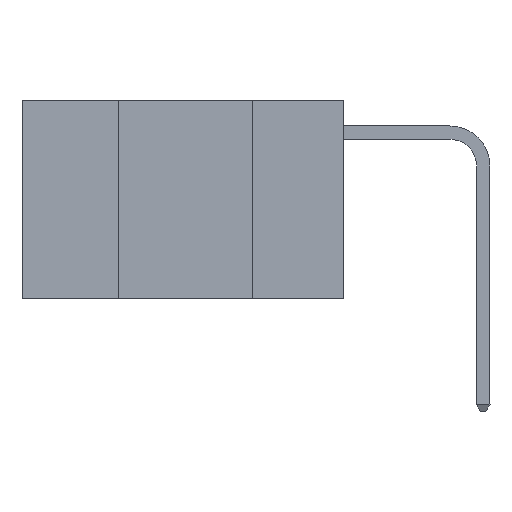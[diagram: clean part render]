
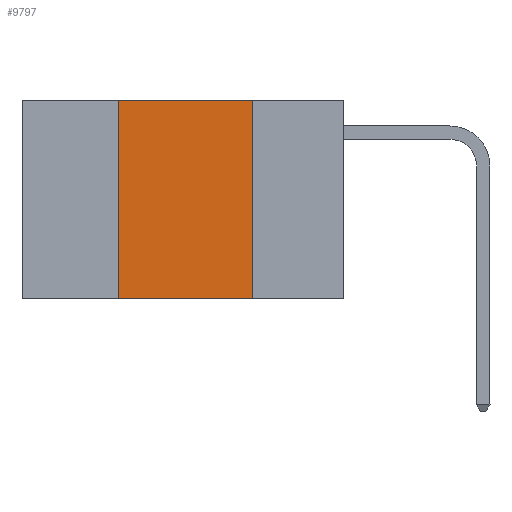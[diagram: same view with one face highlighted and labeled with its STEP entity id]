
A CAD part, left-side view. The second image highlights one B-rep face of the part: STEP entity #9797.
In plain terms, the highlighted planar face has unit normal (-1, 0, 0).
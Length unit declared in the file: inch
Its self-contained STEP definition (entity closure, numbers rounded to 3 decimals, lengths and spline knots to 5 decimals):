
#2934 = VECTOR ( 'NONE', #3183, 39.37008 ) ;
#3183 = DIRECTION ( 'NONE',  ( 0., 0., -1. ) ) ;
#4723 = ORIENTED_EDGE ( 'NONE', *, *, #18762, .F. ) ;
#4965 = ORIENTED_EDGE ( 'NONE', *, *, #8023, .F. ) ;
#5077 = CARTESIAN_POINT ( 'NONE',  ( 0., 0.6, -0.37 ) ) ;
#5193 = DIRECTION ( 'NONE',  ( 1., 0., 0. ) ) ;
#6583 = VECTOR ( 'NONE', #21248, 39.37008 ) ;
#6912 = LINE ( 'NONE', #15313, #2934 ) ;
#7057 = EDGE_LOOP ( 'NONE', ( #4965, #4723, #12502, #15776 ) ) ;
#7082 = CARTESIAN_POINT ( 'NONE',  ( 0., 0.17, 0. ) ) ;
#7115 = LINE ( 'NONE', #5077, #9267 ) ;
#7682 = CARTESIAN_POINT ( 'NONE',  ( 0., 0.42, -0.37 ) ) ;
#8023 = EDGE_CURVE ( 'NONE', #11243, #10568, #6912, .T. ) ;
#8768 = VECTOR ( 'NONE', #11444, 39.37008 ) ;
#9267 = VECTOR ( 'NONE', #17436, 39.37008 ) ;
#9797 = ADVANCED_FACE ( 'NONE', ( #10066 ), #20735, .F. ) ;
#10066 = FACE_OUTER_BOUND ( 'NONE', #7057, .T. ) ;
#10274 = LINE ( 'NONE', #11963, #6583 ) ;
#10568 = VERTEX_POINT ( 'NONE', #14858 ) ;
#11216 = CARTESIAN_POINT ( 'NONE',  ( 0., 0.6, 0. ) ) ;
#11243 = VERTEX_POINT ( 'NONE', #7082 ) ;
#11444 = DIRECTION ( 'NONE',  ( 0., -1., 0. ) ) ;
#11963 = CARTESIAN_POINT ( 'NONE',  ( 0., 0.42, 0. ) ) ;
#12502 = ORIENTED_EDGE ( 'NONE', *, *, #19343, .F. ) ;
#12954 = VERTEX_POINT ( 'NONE', #14923 ) ;
#13129 = AXIS2_PLACEMENT_3D ( 'NONE', #22220, #5193, #17220 ) ;
#13948 = EDGE_CURVE ( 'NONE', #18340, #10568, #7115, .T. ) ;
#14858 = CARTESIAN_POINT ( 'NONE',  ( 0., 0.17, -0.37 ) ) ;
#14923 = CARTESIAN_POINT ( 'NONE',  ( 0., 0.42, 0. ) ) ;
#15313 = CARTESIAN_POINT ( 'NONE',  ( 0., 0.17, 0. ) ) ;
#15776 = ORIENTED_EDGE ( 'NONE', *, *, #13948, .T. ) ;
#17220 = DIRECTION ( 'NONE',  ( 0., 0., -1. ) ) ;
#17436 = DIRECTION ( 'NONE',  ( 0., -1., 0. ) ) ;
#18340 = VERTEX_POINT ( 'NONE', #7682 ) ;
#18762 = EDGE_CURVE ( 'NONE', #12954, #11243, #21898, .T. ) ;
#19343 = EDGE_CURVE ( 'NONE', #18340, #12954, #10274, .T. ) ;
#20735 = PLANE ( 'NONE',  #13129 ) ;
#21248 = DIRECTION ( 'NONE',  ( 0., 0., 1. ) ) ;
#21898 = LINE ( 'NONE', #11216, #8768 ) ;
#22220 = CARTESIAN_POINT ( 'NONE',  ( 0., 0.6, 0. ) ) ;
